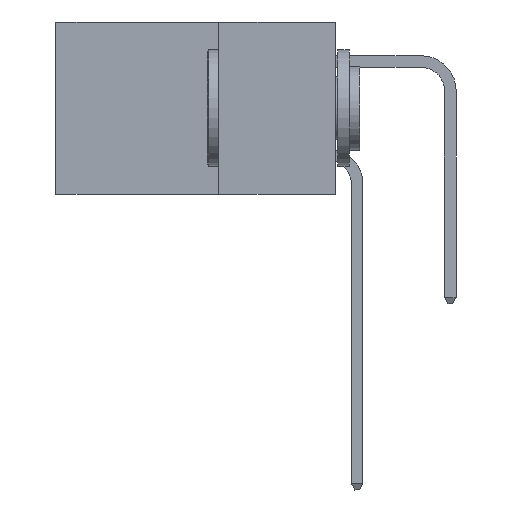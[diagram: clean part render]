
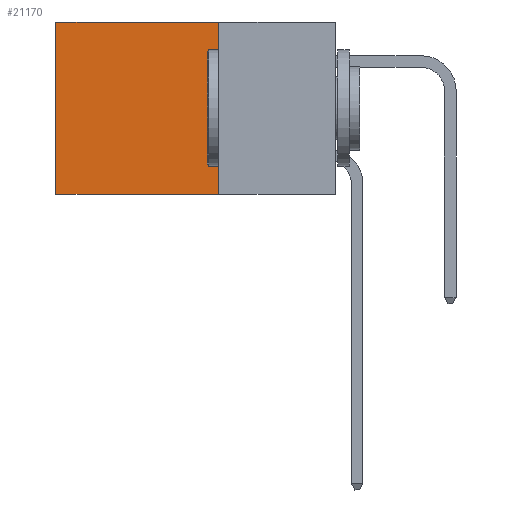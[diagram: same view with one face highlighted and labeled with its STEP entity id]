
A CAD part, left-side view. The second image highlights one B-rep face of the part: STEP entity #21170.
In plain terms, the highlighted planar face has unit normal (-1, 0, 0).
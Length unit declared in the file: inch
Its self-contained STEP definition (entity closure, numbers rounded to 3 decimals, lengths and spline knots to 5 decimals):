
#266 = VERTEX_POINT ( 'NONE', #1171 ) ;
#1171 = CARTESIAN_POINT ( 'NONE',  ( 0.2875, 0.6, 0. ) ) ;
#1376 = CARTESIAN_POINT ( 'NONE',  ( 0.2875, 0.25, 0. ) ) ;
#1498 = EDGE_CURVE ( 'NONE', #18305, #15157, #4382, .T. ) ;
#2374 = LINE ( 'NONE', #9906, #6565 ) ;
#2647 = CARTESIAN_POINT ( 'NONE',  ( 0.2875, 0.6, -0.37 ) ) ;
#4382 = LINE ( 'NONE', #1376, #16006 ) ;
#5126 = CARTESIAN_POINT ( 'NONE',  ( 0.2875, 0.25, 0. ) ) ;
#5257 = DIRECTION ( 'NONE',  ( 0., 0., -1. ) ) ;
#5293 = DIRECTION ( 'NONE',  ( 1., 0., 0. ) ) ;
#6327 = FACE_OUTER_BOUND ( 'NONE', #23046, .T. ) ;
#6565 = VECTOR ( 'NONE', #14021, 39.37008 ) ;
#9414 = CARTESIAN_POINT ( 'NONE',  ( 0.2875, 0.25, -0.37 ) ) ;
#9906 = CARTESIAN_POINT ( 'NONE',  ( 0.2875, 0.25, -0.37 ) ) ;
#10766 = VECTOR ( 'NONE', #25326, 39.37008 ) ;
#11433 = CARTESIAN_POINT ( 'NONE',  ( 0.2875, 0.6, 0. ) ) ;
#12506 = EDGE_CURVE ( 'NONE', #15157, #14544, #2374, .T. ) ;
#14021 = DIRECTION ( 'NONE',  ( 0., 1., 0. ) ) ;
#14544 = VERTEX_POINT ( 'NONE', #2647 ) ;
#14549 = VECTOR ( 'NONE', #19009, 39.37008 ) ;
#15157 = VERTEX_POINT ( 'NONE', #9414 ) ;
#15226 = LINE ( 'NONE', #25245, #14549 ) ;
#15569 = PLANE ( 'NONE',  #26678 ) ;
#16006 = VECTOR ( 'NONE', #5257, 39.37008 ) ;
#16142 = EDGE_CURVE ( 'NONE', #18305, #266, #15226, .T. ) ;
#16450 = ORIENTED_EDGE ( 'NONE', *, *, #12506, .F. ) ;
#17455 = ORIENTED_EDGE ( 'NONE', *, *, #16142, .T. ) ;
#18174 = CARTESIAN_POINT ( 'NONE',  ( 0.2875, 0.25, 0. ) ) ;
#18305 = VERTEX_POINT ( 'NONE', #18174 ) ;
#19009 = DIRECTION ( 'NONE',  ( 0., 1., 0. ) ) ;
#21170 = ADVANCED_FACE ( 'NONE', ( #6327 ), #15569, .F. ) ;
#21796 = LINE ( 'NONE', #11433, #10766 ) ;
#22599 = ORIENTED_EDGE ( 'NONE', *, *, #1498, .F. ) ;
#23046 = EDGE_LOOP ( 'NONE', ( #24988, #16450, #22599, #17455 ) ) ;
#23346 = EDGE_CURVE ( 'NONE', #266, #14544, #21796, .T. ) ;
#23784 = DIRECTION ( 'NONE',  ( 0., 0., -1. ) ) ;
#24988 = ORIENTED_EDGE ( 'NONE', *, *, #23346, .T. ) ;
#25245 = CARTESIAN_POINT ( 'NONE',  ( 0.2875, 0.25, 0. ) ) ;
#25326 = DIRECTION ( 'NONE',  ( 0., 0., -1. ) ) ;
#26678 = AXIS2_PLACEMENT_3D ( 'NONE', #5126, #5293, #23784 ) ;
